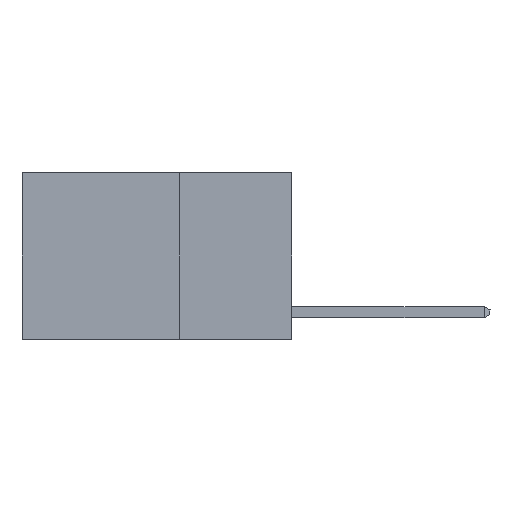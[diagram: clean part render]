
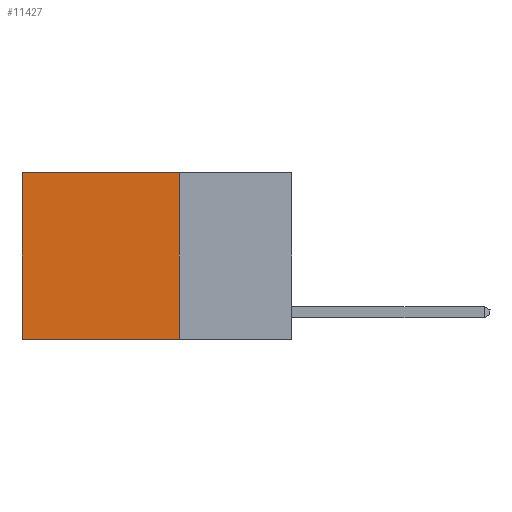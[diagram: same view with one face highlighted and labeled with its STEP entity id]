
A CAD part, left-side view. The second image highlights one B-rep face of the part: STEP entity #11427.
In plain terms, the highlighted planar face has unit normal (-1, 0, 0).
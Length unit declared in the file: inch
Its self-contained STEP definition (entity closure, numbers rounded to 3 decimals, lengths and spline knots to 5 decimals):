
#131 = VERTEX_POINT ( 'NONE', #10411 ) ;
#411 = FACE_OUTER_BOUND ( 'NONE', #11428, .T. ) ;
#689 = ORIENTED_EDGE ( 'NONE', *, *, #6576, .T. ) ;
#761 = CARTESIAN_POINT ( 'NONE',  ( 0.2625, 0.25, -0.37 ) ) ;
#1508 = LINE ( 'NONE', #2303, #7010 ) ;
#1553 = VECTOR ( 'NONE', #6926, 39.37008 ) ;
#1887 = VERTEX_POINT ( 'NONE', #12371 ) ;
#1931 = EDGE_CURVE ( 'NONE', #131, #3586, #7167, .T. ) ;
#2303 = CARTESIAN_POINT ( 'NONE',  ( 0.2625, 0.25, 0. ) ) ;
#3570 = VECTOR ( 'NONE', #5626, 39.37008 ) ;
#3586 = VERTEX_POINT ( 'NONE', #11313 ) ;
#4324 = LINE ( 'NONE', #13901, #1553 ) ;
#4449 = VECTOR ( 'NONE', #7784, 39.37008 ) ;
#4825 = DIRECTION ( 'NONE',  ( 1., 0., 0. ) ) ;
#4894 = ORIENTED_EDGE ( 'NONE', *, *, #14752, .F. ) ;
#5626 = DIRECTION ( 'NONE',  ( 0., 0., -1. ) ) ;
#6576 = EDGE_CURVE ( 'NONE', #1887, #3586, #4324, .T. ) ;
#6926 = DIRECTION ( 'NONE',  ( 0., 0., -1. ) ) ;
#7010 = VECTOR ( 'NONE', #10452, 39.37008 ) ;
#7103 = ORIENTED_EDGE ( 'NONE', *, *, #1931, .F. ) ;
#7167 = LINE ( 'NONE', #761, #4449 ) ;
#7784 = DIRECTION ( 'NONE',  ( 0., 1., 0. ) ) ;
#8586 = CARTESIAN_POINT ( 'NONE',  ( 0.2625, 0.25, 0. ) ) ;
#9454 = CARTESIAN_POINT ( 'NONE',  ( 0.2625, 0.25, 0. ) ) ;
#9766 = LINE ( 'NONE', #11506, #3570 ) ;
#10411 = CARTESIAN_POINT ( 'NONE',  ( 0.2625, 0.25, -0.37 ) ) ;
#10452 = DIRECTION ( 'NONE',  ( 0., 1., 0. ) ) ;
#11313 = CARTESIAN_POINT ( 'NONE',  ( 0.2625, 0.6, -0.37 ) ) ;
#11427 = ADVANCED_FACE ( 'NONE', ( #411 ), #14094, .F. ) ;
#11428 = EDGE_LOOP ( 'NONE', ( #689, #7103, #4894, #14607 ) ) ;
#11506 = CARTESIAN_POINT ( 'NONE',  ( 0.2625, 0.25, 0. ) ) ;
#11750 = AXIS2_PLACEMENT_3D ( 'NONE', #9454, #4825, #12994 ) ;
#12371 = CARTESIAN_POINT ( 'NONE',  ( 0.2625, 0.6, 0. ) ) ;
#12540 = VERTEX_POINT ( 'NONE', #8586 ) ;
#12947 = EDGE_CURVE ( 'NONE', #12540, #1887, #1508, .T. ) ;
#12994 = DIRECTION ( 'NONE',  ( 0., 0., -1. ) ) ;
#13901 = CARTESIAN_POINT ( 'NONE',  ( 0.2625, 0.6, 0. ) ) ;
#14094 = PLANE ( 'NONE',  #11750 ) ;
#14607 = ORIENTED_EDGE ( 'NONE', *, *, #12947, .T. ) ;
#14752 = EDGE_CURVE ( 'NONE', #12540, #131, #9766, .T. ) ;
